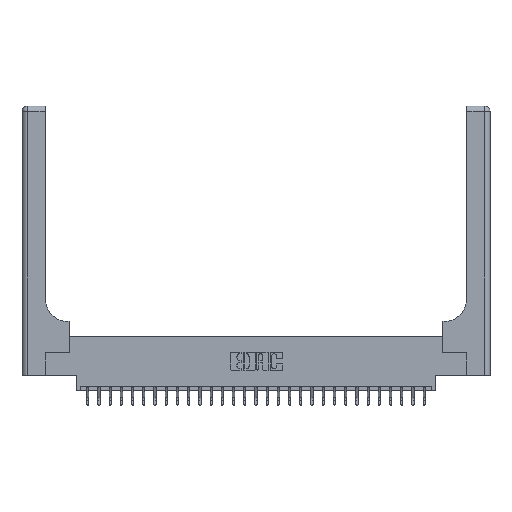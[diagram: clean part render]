
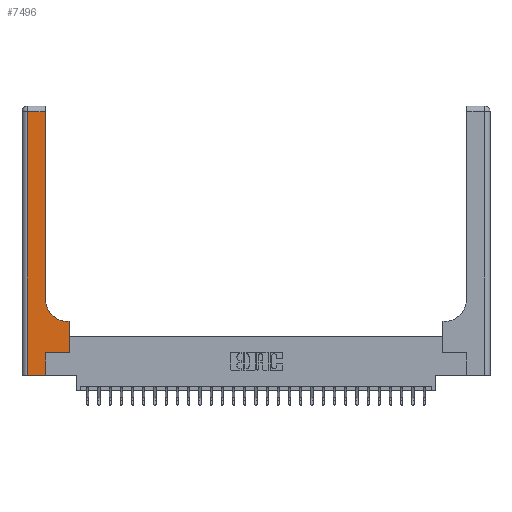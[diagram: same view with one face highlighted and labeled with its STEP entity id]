
A CAD part, top view. The second image highlights one B-rep face of the part: STEP entity #7496.
In plain terms, the highlighted planar face has unit normal (0, 0, 1).
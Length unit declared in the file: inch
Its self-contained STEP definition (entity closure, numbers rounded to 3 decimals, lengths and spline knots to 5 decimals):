
#305 = AXIS2_PLACEMENT_3D ( 'NONE', #11741, #18111, #5486 ) ;
#316 = CARTESIAN_POINT ( 'NONE',  ( 0.265, 0.25, 0.37 ) ) ;
#1153 = ORIENTED_EDGE ( 'NONE', *, *, #22932, .T. ) ;
#1165 = DIRECTION ( 'NONE',  ( 0., 0., -1. ) ) ;
#2436 = CARTESIAN_POINT ( 'NONE',  ( 0., 0., 0.37 ) ) ;
#2573 = CARTESIAN_POINT ( 'NONE',  ( 0.26, 3., 0.37 ) ) ;
#3556 = EDGE_CURVE ( 'NONE', #4664, #13407, #20840, .T. ) ;
#3743 = LINE ( 'NONE', #12150, #25447 ) ;
#4540 = VECTOR ( 'NONE', #25738, 39.37008 ) ;
#4664 = VERTEX_POINT ( 'NONE', #15274 ) ;
#5486 = DIRECTION ( 'NONE',  ( -1., 0., 0. ) ) ;
#6494 = DIRECTION ( 'NONE',  ( -1., 0., 0. ) ) ;
#6692 = DIRECTION ( 'NONE',  ( 0., -1., 0. ) ) ;
#7052 = EDGE_CURVE ( 'NONE', #23890, #20263, #17385, .T. ) ;
#7168 = VERTEX_POINT ( 'NONE', #12861 ) ;
#7292 = ORIENTED_EDGE ( 'NONE', *, *, #18050, .T. ) ;
#7380 = DIRECTION ( 'NONE',  ( -1., 0., 0. ) ) ;
#7496 = ADVANCED_FACE ( 'NONE', ( #27128 ), #22229, .F. ) ;
#7789 = ORIENTED_EDGE ( 'NONE', *, *, #16620, .T. ) ;
#8948 = ORIENTED_EDGE ( 'NONE', *, *, #3556, .T. ) ;
#9393 = EDGE_CURVE ( 'NONE', #13407, #22148, #25369, .T. ) ;
#9999 = DIRECTION ( 'NONE',  ( 0., 1., 0. ) ) ;
#10839 = VECTOR ( 'NONE', #21628, 39.37008 ) ;
#11531 = CARTESIAN_POINT ( 'NONE',  ( 0.26, 0.6, 0.37 ) ) ;
#11741 = CARTESIAN_POINT ( 'NONE',  ( 0., 3., 0.37 ) ) ;
#11968 = CIRCLE ( 'NONE', #25346, 0.25 ) ;
#12150 = CARTESIAN_POINT ( 'NONE',  ( 0.528, 0.25, 0.37 ) ) ;
#12861 = CARTESIAN_POINT ( 'NONE',  ( 0.528, 0.6, 0.37 ) ) ;
#12895 = ORIENTED_EDGE ( 'NONE', *, *, #16136, .T. ) ;
#12930 = ORIENTED_EDGE ( 'NONE', *, *, #9393, .T. ) ;
#13301 = VERTEX_POINT ( 'NONE', #15411 ) ;
#13407 = VERTEX_POINT ( 'NONE', #20097 ) ;
#13810 = CARTESIAN_POINT ( 'NONE',  ( 0.51, 0.85, 0.37 ) ) ;
#14274 = CARTESIAN_POINT ( 'NONE',  ( 0.528, 0.25, 0.37 ) ) ;
#15072 = DIRECTION ( 'NONE',  ( 1., 0., 0. ) ) ;
#15193 = VECTOR ( 'NONE', #7380, 39.37008 ) ;
#15274 = CARTESIAN_POINT ( 'NONE',  ( 0.26, 2.94, 0.37 ) ) ;
#15411 = CARTESIAN_POINT ( 'NONE',  ( 0.51, 0.6, 0.37 ) ) ;
#15875 = LINE ( 'NONE', #11531, #15193 ) ;
#15944 = DIRECTION ( 'NONE',  ( 1., 0., 0. ) ) ;
#16107 = VECTOR ( 'NONE', #15072, 39.37008 ) ;
#16136 = EDGE_CURVE ( 'NONE', #7168, #13301, #15875, .T. ) ;
#16424 = LINE ( 'NONE', #2573, #4540 ) ;
#16620 = EDGE_CURVE ( 'NONE', #16970, #23890, #21402, .T. ) ;
#16682 = VERTEX_POINT ( 'NONE', #25997 ) ;
#16764 = CARTESIAN_POINT ( 'NONE',  ( 0.265, 0.25, 0.37 ) ) ;
#16970 = VERTEX_POINT ( 'NONE', #26696 ) ;
#17013 = CARTESIAN_POINT ( 'NONE',  ( 0., 2.94, 0.37 ) ) ;
#17045 = EDGE_LOOP ( 'NONE', ( #7292, #8948, #12930, #1153, #7789, #17402, #18361, #12895, #27125 ) ) ;
#17385 = LINE ( 'NONE', #16764, #22285 ) ;
#17402 = ORIENTED_EDGE ( 'NONE', *, *, #7052, .T. ) ;
#18050 = EDGE_CURVE ( 'NONE', #16682, #4664, #16424, .T. ) ;
#18111 = DIRECTION ( 'NONE',  ( 0., 0., -1. ) ) ;
#18361 = ORIENTED_EDGE ( 'NONE', *, *, #25573, .T. ) ;
#19532 = CARTESIAN_POINT ( 'NONE',  ( 0.265, 0., 0.37 ) ) ;
#19849 = VECTOR ( 'NONE', #6692, 39.37008 ) ;
#20097 = CARTESIAN_POINT ( 'NONE',  ( 0.06, 2.94, 0.37 ) ) ;
#20263 = VERTEX_POINT ( 'NONE', #14274 ) ;
#20840 = LINE ( 'NONE', #17013, #25724 ) ;
#21402 = LINE ( 'NONE', #19532, #10839 ) ;
#21628 = DIRECTION ( 'NONE',  ( 0., 1., 0. ) ) ;
#22148 = VERTEX_POINT ( 'NONE', #24728 ) ;
#22229 = PLANE ( 'NONE',  #305 ) ;
#22285 = VECTOR ( 'NONE', #27148, 39.37008 ) ;
#22335 = LINE ( 'NONE', #2436, #16107 ) ;
#22932 = EDGE_CURVE ( 'NONE', #22148, #16970, #22335, .T. ) ;
#23413 = CARTESIAN_POINT ( 'NONE',  ( 0.06, 3., 0.37 ) ) ;
#23890 = VERTEX_POINT ( 'NONE', #316 ) ;
#24728 = CARTESIAN_POINT ( 'NONE',  ( 0.06, 0., 0.37 ) ) ;
#25346 = AXIS2_PLACEMENT_3D ( 'NONE', #13810, #1165, #15944 ) ;
#25369 = LINE ( 'NONE', #23413, #19849 ) ;
#25447 = VECTOR ( 'NONE', #9999, 39.37008 ) ;
#25573 = EDGE_CURVE ( 'NONE', #20263, #7168, #3743, .T. ) ;
#25724 = VECTOR ( 'NONE', #6494, 39.37008 ) ;
#25738 = DIRECTION ( 'NONE',  ( 0., 1., 0. ) ) ;
#25973 = EDGE_CURVE ( 'NONE', #13301, #16682, #11968, .T. ) ;
#25997 = CARTESIAN_POINT ( 'NONE',  ( 0.26, 0.85, 0.37 ) ) ;
#26696 = CARTESIAN_POINT ( 'NONE',  ( 0.265, 0., 0.37 ) ) ;
#27125 = ORIENTED_EDGE ( 'NONE', *, *, #25973, .T. ) ;
#27128 = FACE_OUTER_BOUND ( 'NONE', #17045, .T. ) ;
#27148 = DIRECTION ( 'NONE',  ( 1., 0., 0. ) ) ;
